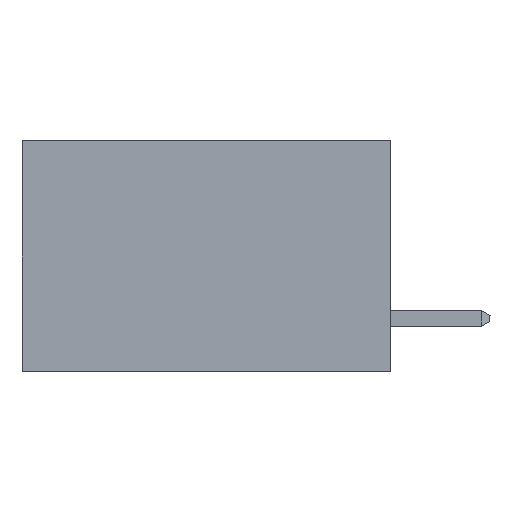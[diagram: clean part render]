
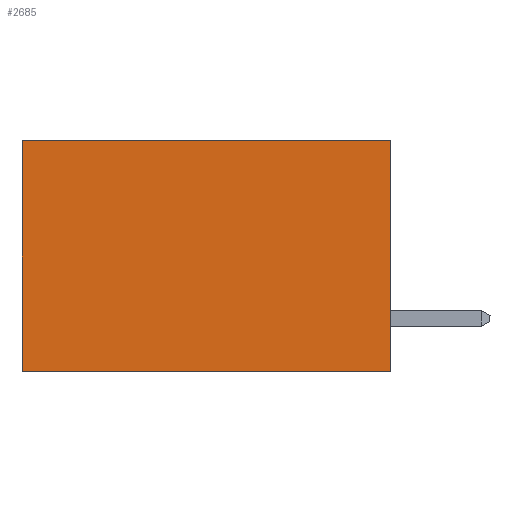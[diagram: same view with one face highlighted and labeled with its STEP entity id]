
A CAD part, left-side view. The second image highlights one B-rep face of the part: STEP entity #2685.
In plain terms, the highlighted planar face has unit normal (-1, 0, 0).
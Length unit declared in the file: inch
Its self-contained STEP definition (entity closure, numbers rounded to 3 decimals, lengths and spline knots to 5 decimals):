
#1464 = EDGE_CURVE ( 'NONE', #1716, #2928, #8723, .T. ) ;
#1530 = EDGE_CURVE ( 'NONE', #8942, #1716, #7580, .T. ) ;
#1716 = VERTEX_POINT ( 'NONE', #6155 ) ;
#2434 = CARTESIAN_POINT ( 'NONE',  ( 0.277, 0.59, -0.37 ) ) ;
#2685 = ADVANCED_FACE ( 'NONE', ( #12866 ), #5875, .F. ) ;
#2928 = VERTEX_POINT ( 'NONE', #2434 ) ;
#3716 = EDGE_LOOP ( 'NONE', ( #4524, #7508, #10703, #7868 ) ) ;
#3772 = DIRECTION ( 'NONE',  ( 0., 0., -1. ) ) ;
#4438 = CARTESIAN_POINT ( 'NONE',  ( 0.277, 0.59, 0. ) ) ;
#4524 = ORIENTED_EDGE ( 'NONE', *, *, #6231, .T. ) ;
#5646 = VECTOR ( 'NONE', #7711, 39.37008 ) ;
#5650 = VECTOR ( 'NONE', #10773, 39.37008 ) ;
#5875 = PLANE ( 'NONE',  #7905 ) ;
#6155 = CARTESIAN_POINT ( 'NONE',  ( 0.277, 0., -0.37 ) ) ;
#6231 = EDGE_CURVE ( 'NONE', #8400, #2928, #8720, .T. ) ;
#7189 = DIRECTION ( 'NONE',  ( 1., 0., 0. ) ) ;
#7508 = ORIENTED_EDGE ( 'NONE', *, *, #1464, .F. ) ;
#7580 = LINE ( 'NONE', #10673, #11102 ) ;
#7711 = DIRECTION ( 'NONE',  ( 0., 0., -1. ) ) ;
#7868 = ORIENTED_EDGE ( 'NONE', *, *, #7954, .T. ) ;
#7905 = AXIS2_PLACEMENT_3D ( 'NONE', #11632, #7189, #13663 ) ;
#7954 = EDGE_CURVE ( 'NONE', #8942, #8400, #13245, .T. ) ;
#8400 = VERTEX_POINT ( 'NONE', #4438 ) ;
#8720 = LINE ( 'NONE', #13036, #5646 ) ;
#8723 = LINE ( 'NONE', #13545, #5650 ) ;
#8942 = VERTEX_POINT ( 'NONE', #13507 ) ;
#9870 = CARTESIAN_POINT ( 'NONE',  ( 0.277, 0., 0. ) ) ;
#10125 = DIRECTION ( 'NONE',  ( 0., 1., 0. ) ) ;
#10380 = VECTOR ( 'NONE', #10125, 39.37008 ) ;
#10673 = CARTESIAN_POINT ( 'NONE',  ( 0.277, 0., -0.37 ) ) ;
#10703 = ORIENTED_EDGE ( 'NONE', *, *, #1530, .F. ) ;
#10773 = DIRECTION ( 'NONE',  ( 0., 1., 0. ) ) ;
#11102 = VECTOR ( 'NONE', #3772, 39.37008 ) ;
#11632 = CARTESIAN_POINT ( 'NONE',  ( 0.277, 0., -0.37 ) ) ;
#12866 = FACE_OUTER_BOUND ( 'NONE', #3716, .T. ) ;
#13036 = CARTESIAN_POINT ( 'NONE',  ( 0.277, 0.59, -0.37 ) ) ;
#13245 = LINE ( 'NONE', #9870, #10380 ) ;
#13507 = CARTESIAN_POINT ( 'NONE',  ( 0.277, 0., 0. ) ) ;
#13545 = CARTESIAN_POINT ( 'NONE',  ( 0.277, 0., -0.37 ) ) ;
#13663 = DIRECTION ( 'NONE',  ( 0., 0., -1. ) ) ;
